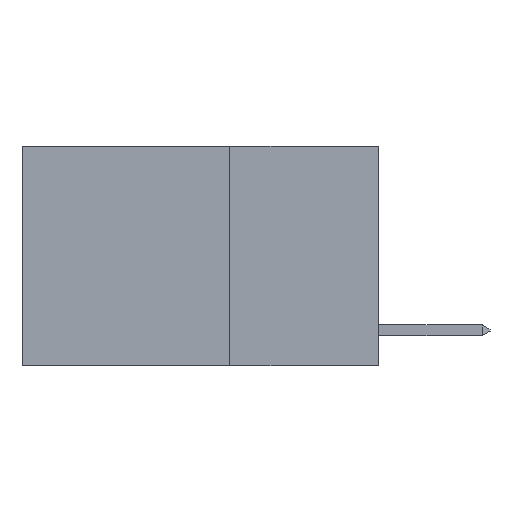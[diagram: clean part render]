
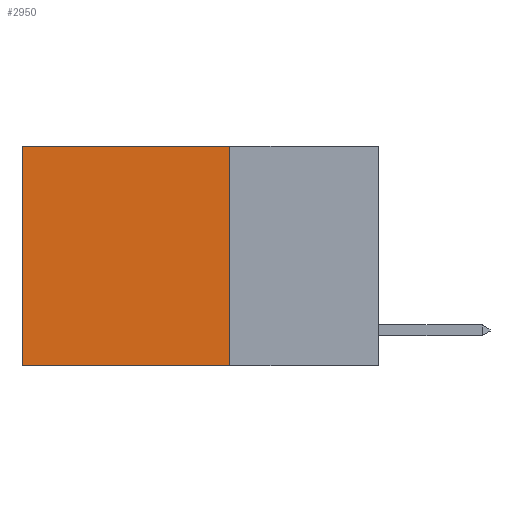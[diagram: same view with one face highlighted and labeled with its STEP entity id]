
A CAD part, left-side view. The second image highlights one B-rep face of the part: STEP entity #2950.
In plain terms, the highlighted planar face has unit normal (-1, 0, 0).
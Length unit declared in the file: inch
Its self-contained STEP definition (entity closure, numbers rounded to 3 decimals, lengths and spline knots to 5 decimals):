
#190 = DIRECTION ( 'NONE',  ( 0., 0., -1. ) ) ;
#212 = DIRECTION ( 'NONE',  ( 0., 1., 0. ) ) ;
#803 = VERTEX_POINT ( 'NONE', #9287 ) ;
#872 = EDGE_LOOP ( 'NONE', ( #3587, #7533, #9092, #1411 ) ) ;
#1196 = VECTOR ( 'NONE', #212, 39.37008 ) ;
#1411 = ORIENTED_EDGE ( 'NONE', *, *, #3448, .T. ) ;
#1907 = EDGE_CURVE ( 'NONE', #803, #4506, #9304, .T. ) ;
#1956 = FACE_OUTER_BOUND ( 'NONE', #872, .T. ) ;
#2708 = LINE ( 'NONE', #9439, #4643 ) ;
#2850 = CARTESIAN_POINT ( 'NONE',  ( 0.2625, 0.25, 0. ) ) ;
#2860 = CARTESIAN_POINT ( 'NONE',  ( 0.2625, 0.25, 0. ) ) ;
#2950 = ADVANCED_FACE ( 'NONE', ( #1956 ), #4214, .F. ) ;
#3363 = CARTESIAN_POINT ( 'NONE',  ( 0.2625, 0.25, 0. ) ) ;
#3448 = EDGE_CURVE ( 'NONE', #4757, #803, #2708, .T. ) ;
#3587 = ORIENTED_EDGE ( 'NONE', *, *, #1907, .T. ) ;
#4214 = PLANE ( 'NONE',  #7906 ) ;
#4506 = VERTEX_POINT ( 'NONE', #8474 ) ;
#4643 = VECTOR ( 'NONE', #5253, 39.37008 ) ;
#4757 = VERTEX_POINT ( 'NONE', #2860 ) ;
#4915 = DIRECTION ( 'NONE',  ( 1., 0., 0. ) ) ;
#4954 = DIRECTION ( 'NONE',  ( 0., 0., -1. ) ) ;
#5253 = DIRECTION ( 'NONE',  ( 0., 1., 0. ) ) ;
#5937 = CARTESIAN_POINT ( 'NONE',  ( 0.2625, 0.25, -0.37 ) ) ;
#6431 = CARTESIAN_POINT ( 'NONE',  ( 0.2625, 0.6, 0. ) ) ;
#7323 = EDGE_CURVE ( 'NONE', #8714, #4506, #7335, .T. ) ;
#7335 = LINE ( 'NONE', #7851, #1196 ) ;
#7522 = VECTOR ( 'NONE', #190, 39.37008 ) ;
#7533 = ORIENTED_EDGE ( 'NONE', *, *, #7323, .F. ) ;
#7638 = EDGE_CURVE ( 'NONE', #4757, #8714, #7857, .T. ) ;
#7851 = CARTESIAN_POINT ( 'NONE',  ( 0.2625, 0.25, -0.37 ) ) ;
#7857 = LINE ( 'NONE', #2850, #9433 ) ;
#7906 = AXIS2_PLACEMENT_3D ( 'NONE', #3363, #4915, #4954 ) ;
#8095 = DIRECTION ( 'NONE',  ( 0., 0., -1. ) ) ;
#8474 = CARTESIAN_POINT ( 'NONE',  ( 0.2625, 0.6, -0.37 ) ) ;
#8714 = VERTEX_POINT ( 'NONE', #5937 ) ;
#9092 = ORIENTED_EDGE ( 'NONE', *, *, #7638, .F. ) ;
#9287 = CARTESIAN_POINT ( 'NONE',  ( 0.2625, 0.6, 0. ) ) ;
#9304 = LINE ( 'NONE', #6431, #7522 ) ;
#9433 = VECTOR ( 'NONE', #8095, 39.37008 ) ;
#9439 = CARTESIAN_POINT ( 'NONE',  ( 0.2625, 0.25, 0. ) ) ;
